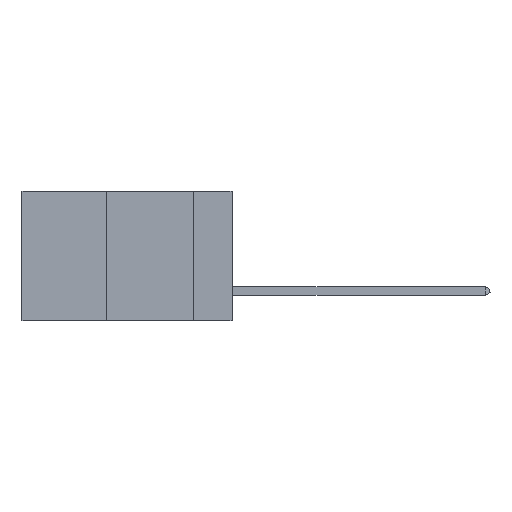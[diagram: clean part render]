
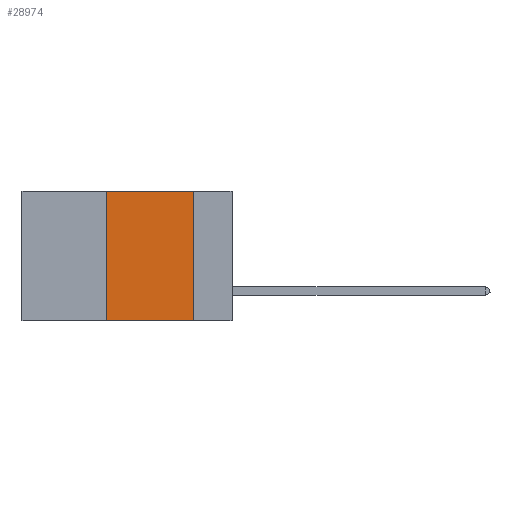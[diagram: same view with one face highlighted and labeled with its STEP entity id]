
A CAD part, left-side view. The second image highlights one B-rep face of the part: STEP entity #28974.
In plain terms, the highlighted planar face has unit normal (-1, 0, 0).
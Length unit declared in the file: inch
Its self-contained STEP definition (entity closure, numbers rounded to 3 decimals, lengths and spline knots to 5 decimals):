
#1481 = CARTESIAN_POINT ( 'NONE',  ( 0., 0.6, -0.37 ) ) ;
#2231 = CARTESIAN_POINT ( 'NONE',  ( 0., 0.11, 0. ) ) ;
#2625 = FACE_OUTER_BOUND ( 'NONE', #8815, .T. ) ;
#2984 = CARTESIAN_POINT ( 'NONE',  ( 0., 0.36, 0. ) ) ;
#3883 = CARTESIAN_POINT ( 'NONE',  ( 0., 0.36, -0.37 ) ) ;
#4688 = DIRECTION ( 'NONE',  ( 0., -1., 0. ) ) ;
#5569 = EDGE_CURVE ( 'NONE', #23857, #13155, #8535, .T. ) ;
#6696 = VERTEX_POINT ( 'NONE', #3883 ) ;
#6787 = CARTESIAN_POINT ( 'NONE',  ( 0., 0.11, -0.37 ) ) ;
#7253 = VECTOR ( 'NONE', #26317, 39.37008 ) ;
#7255 = EDGE_CURVE ( 'NONE', #6696, #23857, #15149, .T. ) ;
#8535 = LINE ( 'NONE', #11705, #13111 ) ;
#8555 = CARTESIAN_POINT ( 'NONE',  ( 0., 0.36, 0. ) ) ;
#8688 = CARTESIAN_POINT ( 'NONE',  ( 0., 0.6, 0. ) ) ;
#8815 = EDGE_LOOP ( 'NONE', ( #25971, #19958, #11887, #14419 ) ) ;
#9394 = CARTESIAN_POINT ( 'NONE',  ( 0., 0.11, 0. ) ) ;
#10977 = DIRECTION ( 'NONE',  ( 0., 0., -1. ) ) ;
#11705 = CARTESIAN_POINT ( 'NONE',  ( 0., 0.6, 0. ) ) ;
#11887 = ORIENTED_EDGE ( 'NONE', *, *, #7255, .F. ) ;
#13111 = VECTOR ( 'NONE', #4688, 39.37008 ) ;
#13155 = VERTEX_POINT ( 'NONE', #2231 ) ;
#14179 = DIRECTION ( 'NONE',  ( 0., 0., -1. ) ) ;
#14419 = ORIENTED_EDGE ( 'NONE', *, *, #20066, .T. ) ;
#15149 = LINE ( 'NONE', #8555, #19689 ) ;
#15340 = DIRECTION ( 'NONE',  ( 0., 0., 1. ) ) ;
#16659 = VECTOR ( 'NONE', #14179, 39.37008 ) ;
#16866 = AXIS2_PLACEMENT_3D ( 'NONE', #8688, #24430, #10977 ) ;
#19689 = VECTOR ( 'NONE', #15340, 39.37008 ) ;
#19814 = LINE ( 'NONE', #9394, #16659 ) ;
#19879 = PLANE ( 'NONE',  #16866 ) ;
#19958 = ORIENTED_EDGE ( 'NONE', *, *, #5569, .F. ) ;
#20066 = EDGE_CURVE ( 'NONE', #6696, #23309, #21315, .T. ) ;
#21315 = LINE ( 'NONE', #1481, #7253 ) ;
#21785 = EDGE_CURVE ( 'NONE', #13155, #23309, #19814, .T. ) ;
#23309 = VERTEX_POINT ( 'NONE', #6787 ) ;
#23857 = VERTEX_POINT ( 'NONE', #2984 ) ;
#24430 = DIRECTION ( 'NONE',  ( 1., 0., 0. ) ) ;
#25971 = ORIENTED_EDGE ( 'NONE', *, *, #21785, .F. ) ;
#26317 = DIRECTION ( 'NONE',  ( 0., -1., 0. ) ) ;
#28974 = ADVANCED_FACE ( 'NONE', ( #2625 ), #19879, .F. ) ;
